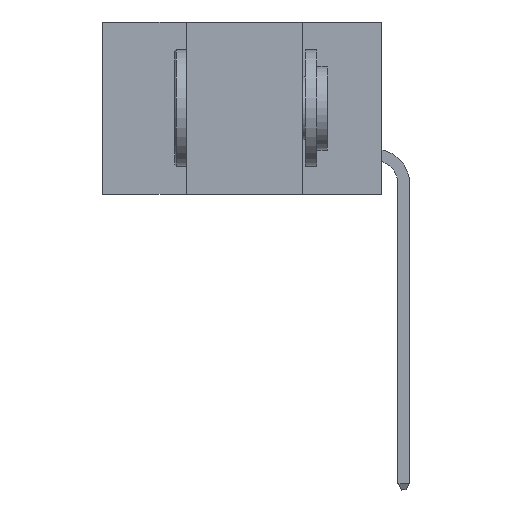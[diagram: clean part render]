
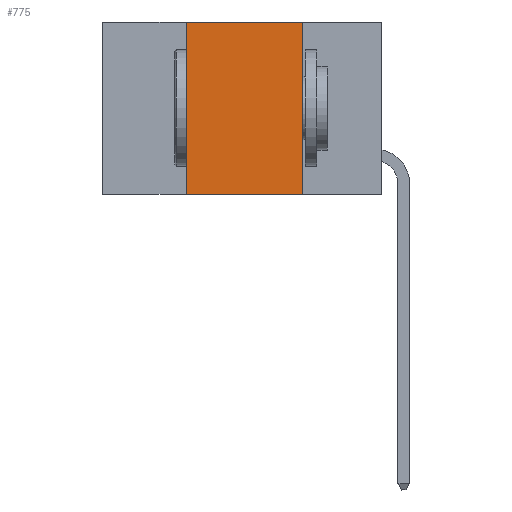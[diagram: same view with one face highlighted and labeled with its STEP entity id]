
A CAD part, left-side view. The second image highlights one B-rep face of the part: STEP entity #775.
In plain terms, the highlighted planar face has unit normal (-1, 0, 0).
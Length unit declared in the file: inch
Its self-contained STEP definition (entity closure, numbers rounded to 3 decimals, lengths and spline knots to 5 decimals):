
#775 = ADVANCED_FACE ( 'NONE', ( #10892 ), #8024, .F. ) ;
#978 = VECTOR ( 'NONE', #16261, 39.37008 ) ;
#1197 = DIRECTION ( 'NONE',  ( 0., -1., 0. ) ) ;
#1263 = CARTESIAN_POINT ( 'NONE',  ( 0., 0.6, 0. ) ) ;
#1310 = VERTEX_POINT ( 'NONE', #4960 ) ;
#1315 = EDGE_CURVE ( 'NONE', #1310, #12784, #4326, .T. ) ;
#1690 = CARTESIAN_POINT ( 'NONE',  ( 0., 0.6, 0. ) ) ;
#2515 = ORIENTED_EDGE ( 'NONE', *, *, #2600, .T. ) ;
#2600 = EDGE_CURVE ( 'NONE', #4963, #12784, #5683, .T. ) ;
#2946 = DIRECTION ( 'NONE',  ( 1., 0., 0. ) ) ;
#3120 = EDGE_LOOP ( 'NONE', ( #16370, #10308, #14298, #2515 ) ) ;
#3491 = CARTESIAN_POINT ( 'NONE',  ( 0., 0.42, 0. ) ) ;
#4326 = LINE ( 'NONE', #15038, #978 ) ;
#4960 = CARTESIAN_POINT ( 'NONE',  ( 0., 0.17, 0. ) ) ;
#4963 = VERTEX_POINT ( 'NONE', #16236 ) ;
#5683 = LINE ( 'NONE', #8818, #15779 ) ;
#6539 = CARTESIAN_POINT ( 'NONE',  ( 0., 0.17, -0.37 ) ) ;
#6676 = AXIS2_PLACEMENT_3D ( 'NONE', #1690, #2946, #13085 ) ;
#7062 = LINE ( 'NONE', #1263, #15578 ) ;
#7602 = DIRECTION ( 'NONE',  ( 0., -1., 0. ) ) ;
#7838 = VECTOR ( 'NONE', #12328, 39.37008 ) ;
#8024 = PLANE ( 'NONE',  #6676 ) ;
#8818 = CARTESIAN_POINT ( 'NONE',  ( 0., 0.6, -0.37 ) ) ;
#10308 = ORIENTED_EDGE ( 'NONE', *, *, #13288, .F. ) ;
#10892 = FACE_OUTER_BOUND ( 'NONE', #3120, .T. ) ;
#11205 = LINE ( 'NONE', #3491, #7838 ) ;
#11591 = CARTESIAN_POINT ( 'NONE',  ( 0., 0.42, 0. ) ) ;
#12151 = VERTEX_POINT ( 'NONE', #11591 ) ;
#12328 = DIRECTION ( 'NONE',  ( 0., 0., 1. ) ) ;
#12784 = VERTEX_POINT ( 'NONE', #6539 ) ;
#13085 = DIRECTION ( 'NONE',  ( 0., 0., -1. ) ) ;
#13288 = EDGE_CURVE ( 'NONE', #12151, #1310, #7062, .T. ) ;
#14004 = EDGE_CURVE ( 'NONE', #4963, #12151, #11205, .T. ) ;
#14298 = ORIENTED_EDGE ( 'NONE', *, *, #14004, .F. ) ;
#15038 = CARTESIAN_POINT ( 'NONE',  ( 0., 0.17, 0. ) ) ;
#15578 = VECTOR ( 'NONE', #7602, 39.37008 ) ;
#15779 = VECTOR ( 'NONE', #1197, 39.37008 ) ;
#16236 = CARTESIAN_POINT ( 'NONE',  ( 0., 0.42, -0.37 ) ) ;
#16261 = DIRECTION ( 'NONE',  ( 0., 0., -1. ) ) ;
#16370 = ORIENTED_EDGE ( 'NONE', *, *, #1315, .F. ) ;
